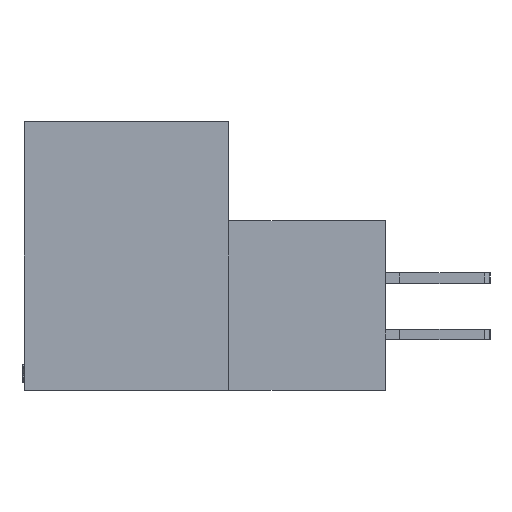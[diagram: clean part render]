
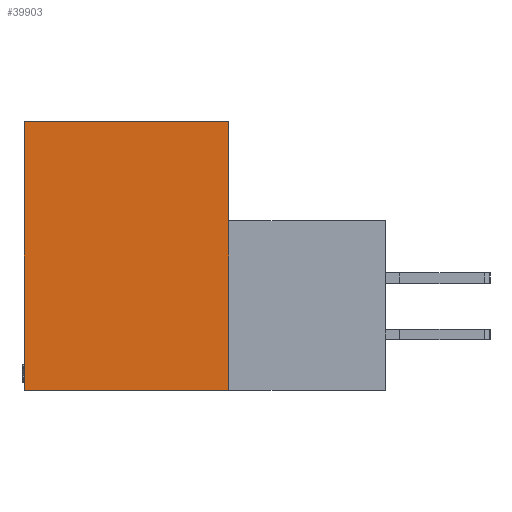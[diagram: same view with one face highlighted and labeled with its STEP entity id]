
A CAD part, left-side view. The second image highlights one B-rep face of the part: STEP entity #39903.
In plain terms, the highlighted planar face has unit normal (-1, 0, 0).
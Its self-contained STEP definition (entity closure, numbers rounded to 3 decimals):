
#3871 = CARTESIAN_POINT ( 'NONE',  ( 0., -8.814, -15.088 ) ) ;
#4711 = AXIS2_PLACEMENT_3D ( 'NONE', #39964, #44104, #47903 ) ;
#4857 = PLANE ( 'NONE',  #4711 ) ;
#7388 = ORIENTED_EDGE ( 'NONE', *, *, #31126, .F. ) ;
#8675 = EDGE_CURVE ( 'NONE', #39524, #12462, #19080, .T. ) ;
#9552 = ORIENTED_EDGE ( 'NONE', *, *, #11075, .F. ) ;
#10731 = EDGE_CURVE ( 'NONE', #12462, #38580, #38662, .T. ) ;
#11075 = EDGE_CURVE ( 'NONE', #18800, #39524, #48521, .T. ) ;
#11618 = DIRECTION ( 'NONE',  ( 0., 1., 0. ) ) ;
#12372 = VECTOR ( 'NONE', #26502, 1000. ) ;
#12462 = VERTEX_POINT ( 'NONE', #41264 ) ;
#17695 = CARTESIAN_POINT ( 'NONE',  ( 0., 0., -15.088 ) ) ;
#18800 = VERTEX_POINT ( 'NONE', #23235 ) ;
#19080 = LINE ( 'NONE', #3871, #36375 ) ;
#22188 = CARTESIAN_POINT ( 'NONE',  ( 0., 11.506, 0. ) ) ;
#23235 = CARTESIAN_POINT ( 'NONE',  ( 0., 0., 0. ) ) ;
#25145 = DIRECTION ( 'NONE',  ( 0., 0., 1. ) ) ;
#25664 = VECTOR ( 'NONE', #49377, 1000. ) ;
#26502 = DIRECTION ( 'NONE',  ( 0., -1., 0. ) ) ;
#29053 = FACE_OUTER_BOUND ( 'NONE', #30538, .T. ) ;
#29318 = CARTESIAN_POINT ( 'NONE',  ( 0., 11.506, -15.088 ) ) ;
#30538 = EDGE_LOOP ( 'NONE', ( #46454, #9552, #7388, #38241 ) ) ;
#31126 = EDGE_CURVE ( 'NONE', #38580, #18800, #45127, .T. ) ;
#36375 = VECTOR ( 'NONE', #11618, 1000. ) ;
#37977 = CARTESIAN_POINT ( 'NONE',  ( 0., 11.506, 0. ) ) ;
#38241 = ORIENTED_EDGE ( 'NONE', *, *, #10731, .F. ) ;
#38580 = VERTEX_POINT ( 'NONE', #37977 ) ;
#38662 = LINE ( 'NONE', #29318, #47350 ) ;
#39524 = VERTEX_POINT ( 'NONE', #17695 ) ;
#39903 = ADVANCED_FACE ( 'NONE', ( #29053 ), #4857, .F. ) ;
#39964 = CARTESIAN_POINT ( 'NONE',  ( 0., 0., 0. ) ) ;
#41264 = CARTESIAN_POINT ( 'NONE',  ( 0., 11.506, -15.088 ) ) ;
#44104 = DIRECTION ( 'NONE',  ( 1., 0., 0. ) ) ;
#45127 = LINE ( 'NONE', #22188, #12372 ) ;
#45214 = CARTESIAN_POINT ( 'NONE',  ( 0., 0., 0. ) ) ;
#46454 = ORIENTED_EDGE ( 'NONE', *, *, #8675, .F. ) ;
#47350 = VECTOR ( 'NONE', #25145, 1000. ) ;
#47903 = DIRECTION ( 'NONE',  ( 0., 0., -1. ) ) ;
#48521 = LINE ( 'NONE', #45214, #25664 ) ;
#49377 = DIRECTION ( 'NONE',  ( 0., 0., -1. ) ) ;
